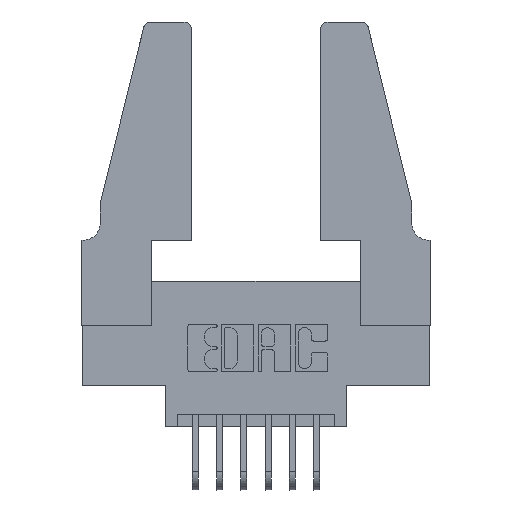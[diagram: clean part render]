
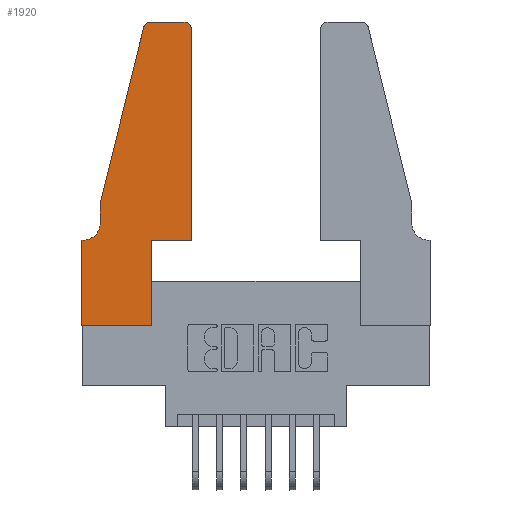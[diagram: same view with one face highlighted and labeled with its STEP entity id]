
A CAD part, top view. The second image highlights one B-rep face of the part: STEP entity #1920.
In plain terms, the highlighted planar face has unit normal (0, 0, 1).
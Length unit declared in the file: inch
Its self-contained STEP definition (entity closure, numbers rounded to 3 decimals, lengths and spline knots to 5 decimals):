
#205 = CARTESIAN_POINT ( 'NONE',  ( 0.0055, 0.42, 0.37 ) ) ;
#256 = VERTEX_POINT ( 'NONE', #5192 ) ;
#303 = EDGE_CURVE ( 'NONE', #7229, #12533, #5334, .T. ) ;
#543 = EDGE_LOOP ( 'NONE', ( #3808, #9286, #11648, #2336, #2037, #1428, #627, #3109, #1946, #563, #6138, #1366 ) ) ;
#563 = ORIENTED_EDGE ( 'NONE', *, *, #303, .T. ) ;
#627 = ORIENTED_EDGE ( 'NONE', *, *, #9152, .T. ) ;
#736 = LINE ( 'NONE', #8553, #2976 ) ;
#776 = CARTESIAN_POINT ( 'NONE',  ( 0.2865, 0.35, 0.37 ) ) ;
#1293 = CARTESIAN_POINT ( 'NONE',  ( 0.25487, 1.22718, 0.37 ) ) ;
#1348 = DIRECTION ( 'NONE',  ( -1., 0., 0. ) ) ;
#1366 = ORIENTED_EDGE ( 'NONE', *, *, #7804, .T. ) ;
#1428 = ORIENTED_EDGE ( 'NONE', *, *, #10578, .T. ) ;
#1456 = VERTEX_POINT ( 'NONE', #9493 ) ;
#1463 = CARTESIAN_POINT ( 'NONE',  ( 0.4505, 0.35, 0.37 ) ) ;
#1651 = DIRECTION ( 'NONE',  ( 0., -1., 0. ) ) ;
#1797 = DIRECTION ( 'NONE',  ( 0., 0., 1. ) ) ;
#1869 = CARTESIAN_POINT ( 'NONE',  ( 0.0055, 0.35, 0.37 ) ) ;
#1920 = ADVANCED_FACE ( 'NONE', ( #11258 ), #11024, .T. ) ;
#1946 = ORIENTED_EDGE ( 'NONE', *, *, #6816, .T. ) ;
#2012 = VECTOR ( 'NONE', #1651, 39.37008 ) ;
#2037 = ORIENTED_EDGE ( 'NONE', *, *, #4322, .T. ) ;
#2260 = VERTEX_POINT ( 'NONE', #6696 ) ;
#2336 = ORIENTED_EDGE ( 'NONE', *, *, #12094, .T. ) ;
#2618 = CARTESIAN_POINT ( 'NONE',  ( 0.284, 1.22, 0.37 ) ) ;
#2635 = VERTEX_POINT ( 'NONE', #1293 ) ;
#2944 = AXIS2_PLACEMENT_3D ( 'NONE', #11059, #10979, #10966 ) ;
#2976 = VECTOR ( 'NONE', #9559, 39.37008 ) ;
#3109 = ORIENTED_EDGE ( 'NONE', *, *, #6960, .T. ) ;
#3599 = CARTESIAN_POINT ( 'NONE',  ( 0., 0., 0.37 ) ) ;
#3689 = DIRECTION ( 'NONE',  ( 1., 0., 0. ) ) ;
#3764 = CARTESIAN_POINT ( 'NONE',  ( 0., 0., 0.37 ) ) ;
#3808 = ORIENTED_EDGE ( 'NONE', *, *, #7839, .T. ) ;
#4300 = LINE ( 'NONE', #1463, #9413 ) ;
#4301 = CARTESIAN_POINT ( 'NONE',  ( 0.0755, 0.42, 0.37 ) ) ;
#4312 = LINE ( 'NONE', #10137, #12164 ) ;
#4322 = EDGE_CURVE ( 'NONE', #8804, #9889, #5565, .T. ) ;
#4591 = CIRCLE ( 'NONE', #6381, 0.03 ) ;
#4916 = VERTEX_POINT ( 'NONE', #10598 ) ;
#5192 = CARTESIAN_POINT ( 'NONE',  ( 0.284, 1.25, 0.37 ) ) ;
#5334 = LINE ( 'NONE', #7474, #7727 ) ;
#5565 = CIRCLE ( 'NONE', #6237, 0.07 ) ;
#5586 = VERTEX_POINT ( 'NONE', #7662 ) ;
#6060 = CARTESIAN_POINT ( 'NONE',  ( 0., 0., 0.37 ) ) ;
#6138 = ORIENTED_EDGE ( 'NONE', *, *, #10998, .T. ) ;
#6165 = CARTESIAN_POINT ( 'NONE',  ( 0.4505, 0.35, 0.37 ) ) ;
#6237 = AXIS2_PLACEMENT_3D ( 'NONE', #205, #7561, #1348 ) ;
#6276 = VECTOR ( 'NONE', #12846, 39.37008 ) ;
#6288 = CARTESIAN_POINT ( 'NONE',  ( 0.0755, 0.5, 0.37 ) ) ;
#6381 = AXIS2_PLACEMENT_3D ( 'NONE', #2618, #9812, #3689 ) ;
#6524 = DIRECTION ( 'NONE',  ( -0.239, -0.971, 0. ) ) ;
#6696 = CARTESIAN_POINT ( 'NONE',  ( 0.2865, 0., 0.37 ) ) ;
#6816 = EDGE_CURVE ( 'NONE', #2260, #7229, #10665, .T. ) ;
#6960 = EDGE_CURVE ( 'NONE', #7911, #2260, #9013, .T. ) ;
#6983 = DIRECTION ( 'NONE',  ( -1., 0., 0. ) ) ;
#7151 = LINE ( 'NONE', #8515, #12333 ) ;
#7229 = VERTEX_POINT ( 'NONE', #776 ) ;
#7474 = CARTESIAN_POINT ( 'NONE',  ( 0.4505, 0.35, 0.37 ) ) ;
#7561 = DIRECTION ( 'NONE',  ( 0., 0., -1. ) ) ;
#7662 = CARTESIAN_POINT ( 'NONE',  ( 0.4505, 1.22, 0.37 ) ) ;
#7727 = VECTOR ( 'NONE', #11071, 39.37008 ) ;
#7804 = EDGE_CURVE ( 'NONE', #5586, #4916, #13326, .T. ) ;
#7839 = EDGE_CURVE ( 'NONE', #4916, #256, #11758, .T. ) ;
#7891 = VECTOR ( 'NONE', #12577, 39.37008 ) ;
#7911 = VERTEX_POINT ( 'NONE', #6060 ) ;
#7984 = CARTESIAN_POINT ( 'NONE',  ( 0.4205, 1.22, 0.37 ) ) ;
#8029 = DIRECTION ( 'NONE',  ( -1., 0., 0. ) ) ;
#8515 = CARTESIAN_POINT ( 'NONE',  ( 0.0755, 0.5, 0.37 ) ) ;
#8553 = CARTESIAN_POINT ( 'NONE',  ( 0.0755, 0.5, 0.37 ) ) ;
#8804 = VERTEX_POINT ( 'NONE', #4301 ) ;
#8990 = VECTOR ( 'NONE', #8029, 39.37008 ) ;
#9013 = LINE ( 'NONE', #3599, #6276 ) ;
#9023 = DIRECTION ( 'NONE',  ( 1., 0., 0. ) ) ;
#9152 = EDGE_CURVE ( 'NONE', #1456, #7911, #12996, .T. ) ;
#9286 = ORIENTED_EDGE ( 'NONE', *, *, #12839, .T. ) ;
#9413 = VECTOR ( 'NONE', #11830, 39.37008 ) ;
#9493 = CARTESIAN_POINT ( 'NONE',  ( 0., 0.35, 0.37 ) ) ;
#9507 = CARTESIAN_POINT ( 'NONE',  ( 0.2865, 0.35, 0.37 ) ) ;
#9559 = DIRECTION ( 'NONE',  ( 0., -1., 0. ) ) ;
#9618 = EDGE_CURVE ( 'NONE', #2635, #12620, #7151, .T. ) ;
#9812 = DIRECTION ( 'NONE',  ( 0., 0., 1. ) ) ;
#9889 = VERTEX_POINT ( 'NONE', #1869 ) ;
#10137 = CARTESIAN_POINT ( 'NONE',  ( 0.0755, 0.35, 0.37 ) ) ;
#10578 = EDGE_CURVE ( 'NONE', #9889, #1456, #4312, .T. ) ;
#10598 = CARTESIAN_POINT ( 'NONE',  ( 0.4205, 1.25, 0.37 ) ) ;
#10665 = LINE ( 'NONE', #9507, #7891 ) ;
#10779 = AXIS2_PLACEMENT_3D ( 'NONE', #7984, #1797, #9023 ) ;
#10966 = DIRECTION ( 'NONE',  ( 1., 0., 0. ) ) ;
#10979 = DIRECTION ( 'NONE',  ( 0., 0., 1. ) ) ;
#10998 = EDGE_CURVE ( 'NONE', #12533, #5586, #4300, .T. ) ;
#11024 = PLANE ( 'NONE',  #2944 ) ;
#11059 = CARTESIAN_POINT ( 'NONE',  ( 0., 0.35, 0.37 ) ) ;
#11071 = DIRECTION ( 'NONE',  ( 1., 0., 0. ) ) ;
#11258 = FACE_OUTER_BOUND ( 'NONE', #543, .T. ) ;
#11648 = ORIENTED_EDGE ( 'NONE', *, *, #9618, .T. ) ;
#11758 = LINE ( 'NONE', #12132, #8990 ) ;
#11830 = DIRECTION ( 'NONE',  ( 0., 1., 0. ) ) ;
#12094 = EDGE_CURVE ( 'NONE', #12620, #8804, #736, .T. ) ;
#12132 = CARTESIAN_POINT ( 'NONE',  ( 0.2605, 1.25, 0.37 ) ) ;
#12164 = VECTOR ( 'NONE', #6983, 39.37008 ) ;
#12333 = VECTOR ( 'NONE', #6524, 39.37008 ) ;
#12533 = VERTEX_POINT ( 'NONE', #6165 ) ;
#12577 = DIRECTION ( 'NONE',  ( 0., 1., 0. ) ) ;
#12620 = VERTEX_POINT ( 'NONE', #6288 ) ;
#12839 = EDGE_CURVE ( 'NONE', #256, #2635, #4591, .T. ) ;
#12846 = DIRECTION ( 'NONE',  ( 1., 0., 0. ) ) ;
#12996 = LINE ( 'NONE', #3764, #2012 ) ;
#13326 = CIRCLE ( 'NONE', #10779, 0.03 ) ;
